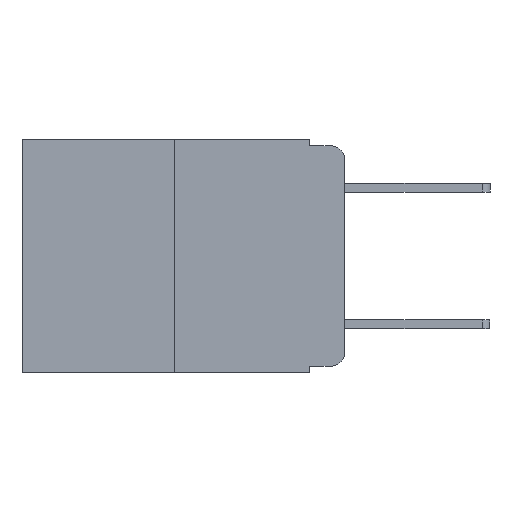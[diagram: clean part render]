
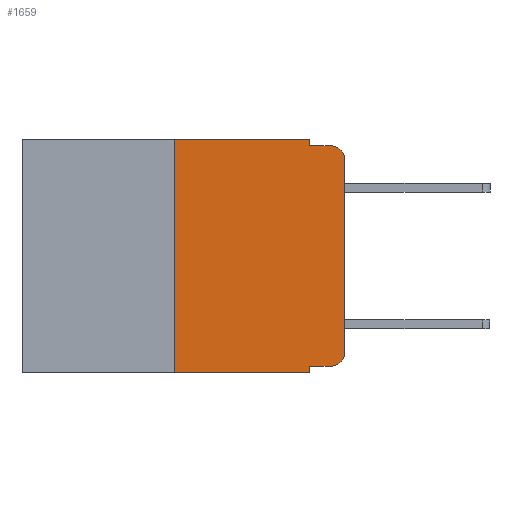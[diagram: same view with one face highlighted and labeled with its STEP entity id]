
A CAD part, left-side view. The second image highlights one B-rep face of the part: STEP entity #1659.
In plain terms, the highlighted planar face has unit normal (-1, 0, 0).
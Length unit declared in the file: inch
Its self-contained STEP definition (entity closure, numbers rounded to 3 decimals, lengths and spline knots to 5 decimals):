
#344 = VECTOR ( 'NONE', #10292, 39.37008 ) ;
#823 = VERTEX_POINT ( 'NONE', #2455 ) ;
#1146 = DIRECTION ( 'NONE',  ( 0., -1., 0. ) ) ;
#1403 = CARTESIAN_POINT ( 'NONE',  ( 0., 0.051, -0.343 ) ) ;
#1659 = ADVANCED_FACE ( 'NONE', ( #12078 ), #7393, .F. ) ;
#1741 = CARTESIAN_POINT ( 'NONE',  ( 0., 0.051, 0. ) ) ;
#1742 = EDGE_CURVE ( 'NONE', #14134, #14482, #10046, .T. ) ;
#2174 = CARTESIAN_POINT ( 'NONE',  ( 0., 0.02, -0.333 ) ) ;
#2254 = LINE ( 'NONE', #11273, #5980 ) ;
#2455 = CARTESIAN_POINT ( 'NONE',  ( 0., 0.051, -0.333 ) ) ;
#2582 = DIRECTION ( 'NONE',  ( 0., 0., -1. ) ) ;
#2616 = DIRECTION ( 'NONE',  ( 0., 0., -1. ) ) ;
#2631 = EDGE_CURVE ( 'NONE', #823, #14134, #7099, .T. ) ;
#2755 = ORIENTED_EDGE ( 'NONE', *, *, #5973, .F. ) ;
#2867 = VERTEX_POINT ( 'NONE', #1403 ) ;
#2872 = LINE ( 'NONE', #8609, #6177 ) ;
#3199 = DIRECTION ( 'NONE',  ( 0., 0., 1. ) ) ;
#3487 = DIRECTION ( 'NONE',  ( -1., 0., 0. ) ) ;
#3514 = EDGE_CURVE ( 'NONE', #823, #2867, #5875, .T. ) ;
#3582 = ORIENTED_EDGE ( 'NONE', *, *, #4415, .F. ) ;
#3742 = VERTEX_POINT ( 'NONE', #11266 ) ;
#4176 = VECTOR ( 'NONE', #4451, 39.37008 ) ;
#4312 = EDGE_CURVE ( 'NONE', #12297, #5487, #10579, .T. ) ;
#4415 = EDGE_CURVE ( 'NONE', #3742, #12297, #5467, .T. ) ;
#4451 = DIRECTION ( 'NONE',  ( 0., -1., 0. ) ) ;
#4630 = ORIENTED_EDGE ( 'NONE', *, *, #1742, .T. ) ;
#4925 = EDGE_LOOP ( 'NONE', ( #13443, #11285, #2755, #9096, #12304, #3582, #13284, #13971, #14972, #4630 ) ) ;
#5005 = CARTESIAN_POINT ( 'NONE',  ( 0., 0.473, 0. ) ) ;
#5037 = CARTESIAN_POINT ( 'NONE',  ( 0., 0.473, -0.343 ) ) ;
#5207 = EDGE_CURVE ( 'NONE', #5487, #6921, #2872, .T. ) ;
#5290 = DIRECTION ( 'NONE',  ( -1., 0., 0. ) ) ;
#5467 = LINE ( 'NONE', #11526, #11074 ) ;
#5487 = VERTEX_POINT ( 'NONE', #1741 ) ;
#5706 = VERTEX_POINT ( 'NONE', #13624 ) ;
#5875 = LINE ( 'NONE', #9667, #11808 ) ;
#5973 = EDGE_CURVE ( 'NONE', #6921, #8005, #7505, .T. ) ;
#5980 = VECTOR ( 'NONE', #3199, 39.37008 ) ;
#5983 = CARTESIAN_POINT ( 'NONE',  ( 0., 0.25, 0. ) ) ;
#6177 = VECTOR ( 'NONE', #2616, 39.37008 ) ;
#6758 = CARTESIAN_POINT ( 'NONE',  ( 0., 0.473, 0. ) ) ;
#6771 = EDGE_CURVE ( 'NONE', #5706, #8005, #8182, .T. ) ;
#6921 = VERTEX_POINT ( 'NONE', #8432 ) ;
#7099 = LINE ( 'NONE', #8097, #344 ) ;
#7393 = PLANE ( 'NONE',  #10168 ) ;
#7505 = LINE ( 'NONE', #7667, #10075 ) ;
#7549 = EDGE_CURVE ( 'NONE', #14482, #5706, #2254, .T. ) ;
#7641 = CARTESIAN_POINT ( 'NONE',  ( 0., 0.02, -0.01 ) ) ;
#7667 = CARTESIAN_POINT ( 'NONE',  ( 0., 0.051, -0.01 ) ) ;
#8005 = VERTEX_POINT ( 'NONE', #7641 ) ;
#8097 = CARTESIAN_POINT ( 'NONE',  ( 0., 0.051, -0.333 ) ) ;
#8182 = CIRCLE ( 'NONE', #9434, 0.02 ) ;
#8253 = DIRECTION ( 'NONE',  ( 0., 0., 1. ) ) ;
#8432 = CARTESIAN_POINT ( 'NONE',  ( 0., 0.051, -0.01 ) ) ;
#8525 = DIRECTION ( 'NONE',  ( 0., 0., -1. ) ) ;
#8609 = CARTESIAN_POINT ( 'NONE',  ( 0., 0.051, 0. ) ) ;
#8757 = EDGE_CURVE ( 'NONE', #3742, #2867, #14849, .T. ) ;
#9096 = ORIENTED_EDGE ( 'NONE', *, *, #5207, .F. ) ;
#9434 = AXIS2_PLACEMENT_3D ( 'NONE', #10430, #3487, #11512 ) ;
#9667 = CARTESIAN_POINT ( 'NONE',  ( 0., 0.051, 0. ) ) ;
#10046 = CIRCLE ( 'NONE', #11086, 0.02 ) ;
#10075 = VECTOR ( 'NONE', #14136, 39.37008 ) ;
#10168 = AXIS2_PLACEMENT_3D ( 'NONE', #5005, #14945, #8525 ) ;
#10292 = DIRECTION ( 'NONE',  ( 0., -1., 0. ) ) ;
#10430 = CARTESIAN_POINT ( 'NONE',  ( 0., 0.02, -0.03 ) ) ;
#10579 = LINE ( 'NONE', #6758, #4176 ) ;
#10805 = CARTESIAN_POINT ( 'NONE',  ( 0., 0., -0.313 ) ) ;
#11074 = VECTOR ( 'NONE', #8253, 39.37008 ) ;
#11086 = AXIS2_PLACEMENT_3D ( 'NONE', #11972, #5290, #13022 ) ;
#11266 = CARTESIAN_POINT ( 'NONE',  ( 0., 0.25, -0.343 ) ) ;
#11273 = CARTESIAN_POINT ( 'NONE',  ( 0., 0., 0. ) ) ;
#11285 = ORIENTED_EDGE ( 'NONE', *, *, #6771, .T. ) ;
#11512 = DIRECTION ( 'NONE',  ( 0., 0., -1. ) ) ;
#11526 = CARTESIAN_POINT ( 'NONE',  ( 0., 0.25, 0. ) ) ;
#11808 = VECTOR ( 'NONE', #2582, 39.37008 ) ;
#11972 = CARTESIAN_POINT ( 'NONE',  ( 0., 0.02, -0.313 ) ) ;
#12023 = VECTOR ( 'NONE', #1146, 39.37008 ) ;
#12078 = FACE_OUTER_BOUND ( 'NONE', #4925, .T. ) ;
#12297 = VERTEX_POINT ( 'NONE', #5983 ) ;
#12304 = ORIENTED_EDGE ( 'NONE', *, *, #4312, .F. ) ;
#13022 = DIRECTION ( 'NONE',  ( 0., 0., -1. ) ) ;
#13284 = ORIENTED_EDGE ( 'NONE', *, *, #8757, .T. ) ;
#13443 = ORIENTED_EDGE ( 'NONE', *, *, #7549, .T. ) ;
#13624 = CARTESIAN_POINT ( 'NONE',  ( 0., 0., -0.03 ) ) ;
#13971 = ORIENTED_EDGE ( 'NONE', *, *, #3514, .F. ) ;
#14134 = VERTEX_POINT ( 'NONE', #2174 ) ;
#14136 = DIRECTION ( 'NONE',  ( 0., -1., 0. ) ) ;
#14482 = VERTEX_POINT ( 'NONE', #10805 ) ;
#14849 = LINE ( 'NONE', #5037, #12023 ) ;
#14945 = DIRECTION ( 'NONE',  ( 1., 0., 0. ) ) ;
#14972 = ORIENTED_EDGE ( 'NONE', *, *, #2631, .T. ) ;
